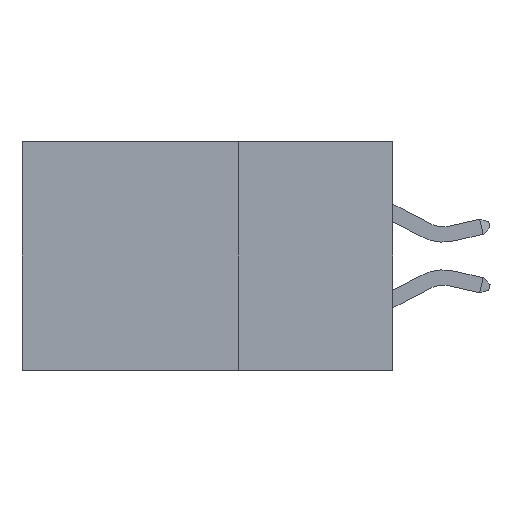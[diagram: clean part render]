
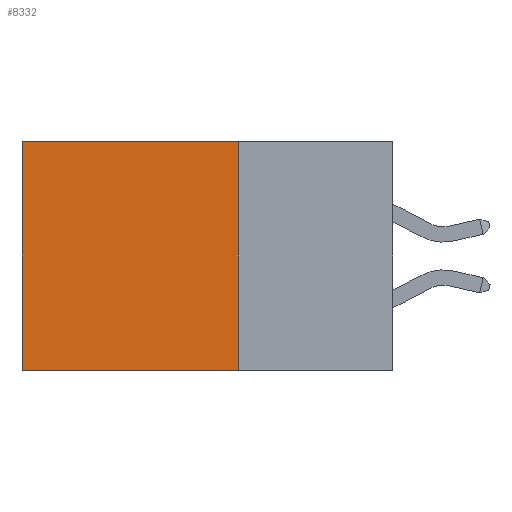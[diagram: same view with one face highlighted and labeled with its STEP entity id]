
A CAD part, left-side view. The second image highlights one B-rep face of the part: STEP entity #8332.
In plain terms, the highlighted planar face has unit normal (-1, 0, 0).
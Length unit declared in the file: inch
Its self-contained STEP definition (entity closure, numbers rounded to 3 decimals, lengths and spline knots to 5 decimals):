
#1713 = VERTEX_POINT ( 'NONE', #12716 ) ;
#1757 = FACE_OUTER_BOUND ( 'NONE', #9457, .T. ) ;
#2355 = EDGE_CURVE ( 'NONE', #13724, #1713, #6113, .T. ) ;
#2442 = DIRECTION ( 'NONE',  ( 0., 0., -1. ) ) ;
#2574 = ORIENTED_EDGE ( 'NONE', *, *, #7625, .T. ) ;
#2826 = VECTOR ( 'NONE', #3142, 39.37008 ) ;
#2953 = DIRECTION ( 'NONE',  ( 1., 0., 0. ) ) ;
#3142 = DIRECTION ( 'NONE',  ( 0., 0., -1. ) ) ;
#3648 = LINE ( 'NONE', #9063, #13154 ) ;
#4770 = EDGE_CURVE ( 'NONE', #15326, #13724, #15098, .T. ) ;
#5504 = CARTESIAN_POINT ( 'NONE',  ( 0.2875, 0.25, 0. ) ) ;
#6113 = LINE ( 'NONE', #10640, #6302 ) ;
#6230 = LINE ( 'NONE', #16283, #17459 ) ;
#6302 = VECTOR ( 'NONE', #16931, 39.37008 ) ;
#6771 = DIRECTION ( 'NONE',  ( 0., 1., 0. ) ) ;
#7625 = EDGE_CURVE ( 'NONE', #15326, #12876, #6230, .T. ) ;
#8077 = ORIENTED_EDGE ( 'NONE', *, *, #8578, .T. ) ;
#8332 = ADVANCED_FACE ( 'NONE', ( #1757 ), #13715, .F. ) ;
#8578 = EDGE_CURVE ( 'NONE', #12876, #1713, #3648, .T. ) ;
#8928 = CARTESIAN_POINT ( 'NONE',  ( 0.2875, 0.25, -0.37 ) ) ;
#9063 = CARTESIAN_POINT ( 'NONE',  ( 0.2875, 0.6, 0. ) ) ;
#9457 = EDGE_LOOP ( 'NONE', ( #8077, #12454, #16037, #2574 ) ) ;
#10640 = CARTESIAN_POINT ( 'NONE',  ( 0.2875, 0.25, -0.37 ) ) ;
#12454 = ORIENTED_EDGE ( 'NONE', *, *, #2355, .F. ) ;
#12716 = CARTESIAN_POINT ( 'NONE',  ( 0.2875, 0.6, -0.37 ) ) ;
#12876 = VERTEX_POINT ( 'NONE', #16856 ) ;
#13154 = VECTOR ( 'NONE', #2442, 39.37008 ) ;
#13715 = PLANE ( 'NONE',  #17090 ) ;
#13724 = VERTEX_POINT ( 'NONE', #8928 ) ;
#15098 = LINE ( 'NONE', #15260, #2826 ) ;
#15260 = CARTESIAN_POINT ( 'NONE',  ( 0.2875, 0.25, 0. ) ) ;
#15326 = VERTEX_POINT ( 'NONE', #15662 ) ;
#15662 = CARTESIAN_POINT ( 'NONE',  ( 0.2875, 0.25, 0. ) ) ;
#16037 = ORIENTED_EDGE ( 'NONE', *, *, #4770, .F. ) ;
#16279 = DIRECTION ( 'NONE',  ( 0., 0., -1. ) ) ;
#16283 = CARTESIAN_POINT ( 'NONE',  ( 0.2875, 0.25, 0. ) ) ;
#16856 = CARTESIAN_POINT ( 'NONE',  ( 0.2875, 0.6, 0. ) ) ;
#16931 = DIRECTION ( 'NONE',  ( 0., 1., 0. ) ) ;
#17090 = AXIS2_PLACEMENT_3D ( 'NONE', #5504, #2953, #16279 ) ;
#17459 = VECTOR ( 'NONE', #6771, 39.37008 ) ;
